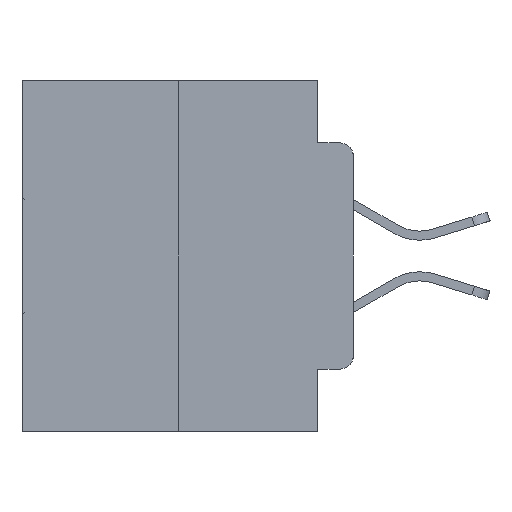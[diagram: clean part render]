
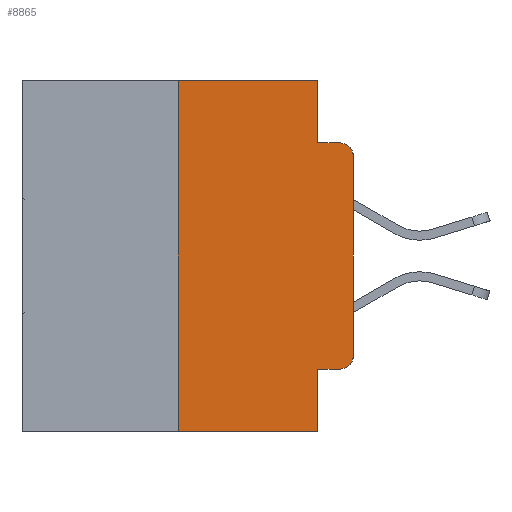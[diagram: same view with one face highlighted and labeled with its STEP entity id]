
A CAD part, left-side view. The second image highlights one B-rep face of the part: STEP entity #8865.
In plain terms, the highlighted planar face has unit normal (-1, 0, 0).
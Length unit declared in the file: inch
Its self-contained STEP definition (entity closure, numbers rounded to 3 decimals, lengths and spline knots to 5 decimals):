
#206 = EDGE_CURVE ( 'NONE', #2833, #6278, #28457, .T. ) ;
#1209 = CARTESIAN_POINT ( 'NONE',  ( 0., 0.051, 0. ) ) ;
#1693 = AXIS2_PLACEMENT_3D ( 'NONE', #25298, #11509, #13993 ) ;
#1973 = ORIENTED_EDGE ( 'NONE', *, *, #5383, .T. ) ;
#2052 = ORIENTED_EDGE ( 'NONE', *, *, #10743, .F. ) ;
#2177 = ORIENTED_EDGE ( 'NONE', *, *, #206, .F. ) ;
#2337 = VERTEX_POINT ( 'NONE', #25653 ) ;
#2691 = CIRCLE ( 'NONE', #1693, 0.02 ) ;
#2833 = VERTEX_POINT ( 'NONE', #23380 ) ;
#2981 = VECTOR ( 'NONE', #4761, 39.37008 ) ;
#3430 = CARTESIAN_POINT ( 'NONE',  ( 0., 0.473, 0. ) ) ;
#3507 = LINE ( 'NONE', #19340, #21211 ) ;
#3607 = EDGE_LOOP ( 'NONE', ( #1973, #21203, #25642, #2177, #15936, #8357, #23615, #2052, #14970, #18918 ) ) ;
#3663 = EDGE_CURVE ( 'NONE', #6278, #14572, #3507, .T. ) ;
#4761 = DIRECTION ( 'NONE',  ( 0., -1., 0. ) ) ;
#5023 = CARTESIAN_POINT ( 'NONE',  ( 0., 0.473, 0. ) ) ;
#5383 = EDGE_CURVE ( 'NONE', #18517, #23937, #7802, .T. ) ;
#5914 = DIRECTION ( 'NONE',  ( -1., 0., 0. ) ) ;
#6278 = VERTEX_POINT ( 'NONE', #28908 ) ;
#6482 = VECTOR ( 'NONE', #27526, 39.37008 ) ;
#6522 = EDGE_CURVE ( 'NONE', #2337, #18517, #2691, .T. ) ;
#6588 = CARTESIAN_POINT ( 'NONE',  ( 0., 0.02, -0.0885 ) ) ;
#6969 = AXIS2_PLACEMENT_3D ( 'NONE', #3430, #8073, #23800 ) ;
#7360 = DIRECTION ( 'NONE',  ( 0., -1., 0. ) ) ;
#7427 = EDGE_CURVE ( 'NONE', #23937, #14572, #29612, .T. ) ;
#7802 = LINE ( 'NONE', #25470, #24751 ) ;
#8025 = CARTESIAN_POINT ( 'NONE',  ( 0., 0.02, -0.1085 ) ) ;
#8073 = DIRECTION ( 'NONE',  ( 1., 0., 0. ) ) ;
#8079 = DIRECTION ( 'NONE',  ( 0., 0., -1. ) ) ;
#8357 = ORIENTED_EDGE ( 'NONE', *, *, #21003, .F. ) ;
#8865 = ADVANCED_FACE ( 'NONE', ( #23121 ), #28683, .F. ) ;
#10516 = EDGE_CURVE ( 'NONE', #24210, #2337, #24621, .T. ) ;
#10743 = EDGE_CURVE ( 'NONE', #24210, #13635, #14497, .T. ) ;
#11509 = DIRECTION ( 'NONE',  ( -1., 0., 0. ) ) ;
#12602 = VECTOR ( 'NONE', #7360, 39.37008 ) ;
#13056 = CARTESIAN_POINT ( 'NONE',  ( 0., 0.473, -0.5 ) ) ;
#13635 = VERTEX_POINT ( 'NONE', #14733 ) ;
#13993 = DIRECTION ( 'NONE',  ( 0., 0., -1. ) ) ;
#14497 = LINE ( 'NONE', #28391, #15930 ) ;
#14572 = VERTEX_POINT ( 'NONE', #6588 ) ;
#14733 = CARTESIAN_POINT ( 'NONE',  ( 0., 0.051, -0.5 ) ) ;
#14959 = CARTESIAN_POINT ( 'NONE',  ( 0., 0.051, -0.4115 ) ) ;
#14970 = ORIENTED_EDGE ( 'NONE', *, *, #10516, .T. ) ;
#15930 = VECTOR ( 'NONE', #8079, 39.37008 ) ;
#15936 = ORIENTED_EDGE ( 'NONE', *, *, #23943, .F. ) ;
#16940 = VECTOR ( 'NONE', #17327, 39.37008 ) ;
#17172 = CARTESIAN_POINT ( 'NONE',  ( 0., 0.25, 0. ) ) ;
#17309 = DIRECTION ( 'NONE',  ( 0., -1., 0. ) ) ;
#17327 = DIRECTION ( 'NONE',  ( 0., 0., -1. ) ) ;
#18517 = VERTEX_POINT ( 'NONE', #24678 ) ;
#18816 = DIRECTION ( 'NONE',  ( 0., 0., 1. ) ) ;
#18918 = ORIENTED_EDGE ( 'NONE', *, *, #6522, .T. ) ;
#19340 = CARTESIAN_POINT ( 'NONE',  ( 0., 0.051, -0.0885 ) ) ;
#21003 = EDGE_CURVE ( 'NONE', #22545, #27839, #25933, .T. ) ;
#21175 = CARTESIAN_POINT ( 'NONE',  ( 0., 0., -0.1085 ) ) ;
#21203 = ORIENTED_EDGE ( 'NONE', *, *, #7427, .T. ) ;
#21211 = VECTOR ( 'NONE', #17309, 39.37008 ) ;
#21217 = EDGE_CURVE ( 'NONE', #22545, #13635, #24860, .T. ) ;
#22545 = VERTEX_POINT ( 'NONE', #27362 ) ;
#23061 = LINE ( 'NONE', #5023, #12602 ) ;
#23121 = FACE_OUTER_BOUND ( 'NONE', #3607, .T. ) ;
#23170 = AXIS2_PLACEMENT_3D ( 'NONE', #8025, #5914, #26238 ) ;
#23310 = CARTESIAN_POINT ( 'NONE',  ( 0., 0.051, -0.4115 ) ) ;
#23380 = CARTESIAN_POINT ( 'NONE',  ( 0., 0.051, 0. ) ) ;
#23615 = ORIENTED_EDGE ( 'NONE', *, *, #21217, .T. ) ;
#23800 = DIRECTION ( 'NONE',  ( 0., 0., -1. ) ) ;
#23937 = VERTEX_POINT ( 'NONE', #21175 ) ;
#23943 = EDGE_CURVE ( 'NONE', #27839, #2833, #23061, .T. ) ;
#24210 = VERTEX_POINT ( 'NONE', #14959 ) ;
#24621 = LINE ( 'NONE', #23310, #2981 ) ;
#24678 = CARTESIAN_POINT ( 'NONE',  ( 0., 0., -0.3915 ) ) ;
#24751 = VECTOR ( 'NONE', #18816, 39.37008 ) ;
#24860 = LINE ( 'NONE', #13056, #6482 ) ;
#25298 = CARTESIAN_POINT ( 'NONE',  ( 0., 0.02, -0.3915 ) ) ;
#25470 = CARTESIAN_POINT ( 'NONE',  ( 0., 0., 0. ) ) ;
#25642 = ORIENTED_EDGE ( 'NONE', *, *, #3663, .F. ) ;
#25653 = CARTESIAN_POINT ( 'NONE',  ( 0., 0.02, -0.4115 ) ) ;
#25933 = LINE ( 'NONE', #17172, #26305 ) ;
#26238 = DIRECTION ( 'NONE',  ( 0., 0., -1. ) ) ;
#26241 = DIRECTION ( 'NONE',  ( 0., 0., 1. ) ) ;
#26305 = VECTOR ( 'NONE', #26241, 39.37008 ) ;
#27362 = CARTESIAN_POINT ( 'NONE',  ( 0., 0.25, -0.5 ) ) ;
#27526 = DIRECTION ( 'NONE',  ( 0., -1., 0. ) ) ;
#27839 = VERTEX_POINT ( 'NONE', #28997 ) ;
#28391 = CARTESIAN_POINT ( 'NONE',  ( 0., 0.051, 0. ) ) ;
#28457 = LINE ( 'NONE', #1209, #16940 ) ;
#28683 = PLANE ( 'NONE',  #6969 ) ;
#28908 = CARTESIAN_POINT ( 'NONE',  ( 0., 0.051, -0.0885 ) ) ;
#28997 = CARTESIAN_POINT ( 'NONE',  ( 0., 0.25, 0. ) ) ;
#29612 = CIRCLE ( 'NONE', #23170, 0.02 ) ;
